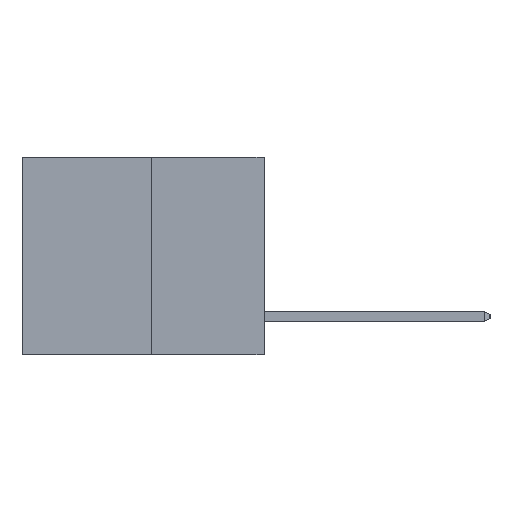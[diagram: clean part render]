
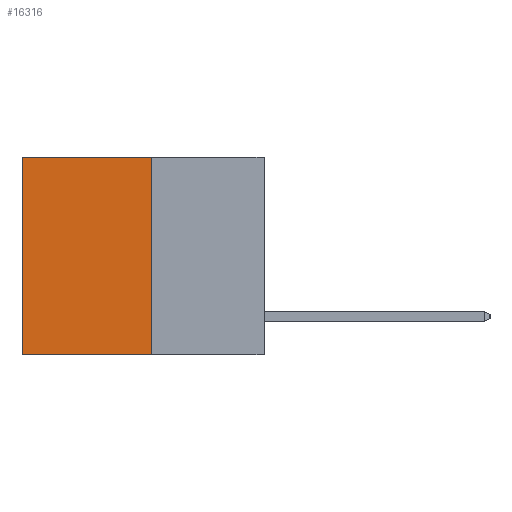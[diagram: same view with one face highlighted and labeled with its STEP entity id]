
A CAD part, left-side view. The second image highlights one B-rep face of the part: STEP entity #16316.
In plain terms, the highlighted planar face has unit normal (-1, 0, 0).
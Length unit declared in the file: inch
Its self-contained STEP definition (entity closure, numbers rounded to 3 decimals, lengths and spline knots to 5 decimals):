
#127 = FACE_OUTER_BOUND ( 'NONE', #22740, .T. ) ;
#225 = PLANE ( 'NONE',  #732 ) ;
#732 = AXIS2_PLACEMENT_3D ( 'NONE', #25045, #8581, #8309 ) ;
#2009 = ORIENTED_EDGE ( 'NONE', *, *, #3513, .T. ) ;
#3513 = EDGE_CURVE ( 'NONE', #22761, #7356, #6599, .T. ) ;
#3958 = VERTEX_POINT ( 'NONE', #27048 ) ;
#4015 = CARTESIAN_POINT ( 'NONE',  ( 0.3165, 0.28, -0.49 ) ) ;
#4290 = CARTESIAN_POINT ( 'NONE',  ( 0.3165, 0.28, -0.49 ) ) ;
#4668 = DIRECTION ( 'NONE',  ( 0., 1., 0. ) ) ;
#6599 = LINE ( 'NONE', #9877, #21972 ) ;
#6981 = CARTESIAN_POINT ( 'NONE',  ( 0.3165, 0.28, -0.49 ) ) ;
#7356 = VERTEX_POINT ( 'NONE', #8000 ) ;
#8000 = CARTESIAN_POINT ( 'NONE',  ( 0.3165, 0.6, -0.49 ) ) ;
#8309 = DIRECTION ( 'NONE',  ( 0., 0., -1. ) ) ;
#8581 = DIRECTION ( 'NONE',  ( 1., 0., 0. ) ) ;
#9877 = CARTESIAN_POINT ( 'NONE',  ( 0.3165, 0.6, -0.49 ) ) ;
#9966 = DIRECTION ( 'NONE',  ( 0., 0., -1. ) ) ;
#10893 = ORIENTED_EDGE ( 'NONE', *, *, #18604, .F. ) ;
#11912 = VECTOR ( 'NONE', #15816, 39.37008 ) ;
#11933 = VECTOR ( 'NONE', #4668, 39.37008 ) ;
#15816 = DIRECTION ( 'NONE',  ( 0., 1., 0. ) ) ;
#16316 = ADVANCED_FACE ( 'NONE', ( #127 ), #225, .F. ) ;
#17008 = EDGE_CURVE ( 'NONE', #3958, #22761, #23025, .T. ) ;
#17466 = LINE ( 'NONE', #4290, #11933 ) ;
#18521 = ORIENTED_EDGE ( 'NONE', *, *, #17008, .T. ) ;
#18604 = EDGE_CURVE ( 'NONE', #20605, #7356, #17466, .T. ) ;
#18983 = LINE ( 'NONE', #6981, #25546 ) ;
#20605 = VERTEX_POINT ( 'NONE', #4015 ) ;
#21243 = DIRECTION ( 'NONE',  ( 0., 0., -1. ) ) ;
#21972 = VECTOR ( 'NONE', #9966, 39.37008 ) ;
#22740 = EDGE_LOOP ( 'NONE', ( #2009, #10893, #27030, #18521 ) ) ;
#22761 = VERTEX_POINT ( 'NONE', #23271 ) ;
#23025 = LINE ( 'NONE', #24298, #11912 ) ;
#23271 = CARTESIAN_POINT ( 'NONE',  ( 0.3165, 0.6, 0. ) ) ;
#24109 = EDGE_CURVE ( 'NONE', #3958, #20605, #18983, .T. ) ;
#24298 = CARTESIAN_POINT ( 'NONE',  ( 0.3165, 0.28, 0. ) ) ;
#25045 = CARTESIAN_POINT ( 'NONE',  ( 0.3165, 0.28, -0.49 ) ) ;
#25546 = VECTOR ( 'NONE', #21243, 39.37008 ) ;
#27030 = ORIENTED_EDGE ( 'NONE', *, *, #24109, .F. ) ;
#27048 = CARTESIAN_POINT ( 'NONE',  ( 0.3165, 0.28, 0. ) ) ;
